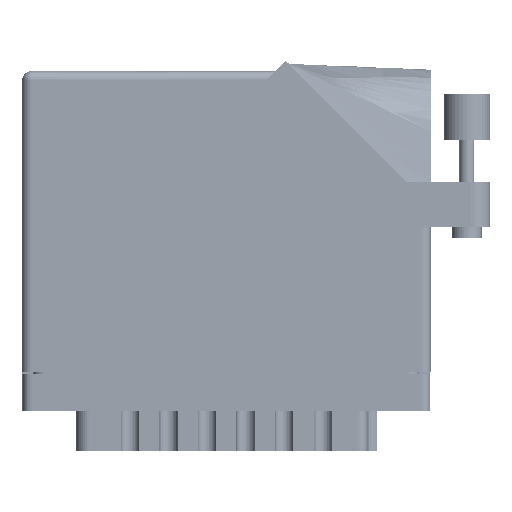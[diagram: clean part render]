
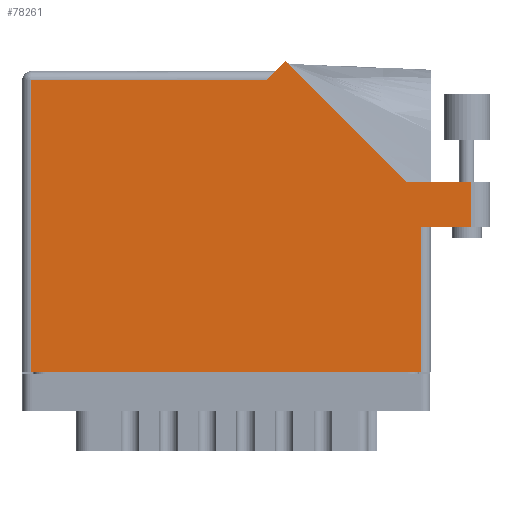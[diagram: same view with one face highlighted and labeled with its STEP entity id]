
A CAD part, front view. The second image highlights one B-rep face of the part: STEP entity #78261.
In plain terms, the highlighted face is planar.
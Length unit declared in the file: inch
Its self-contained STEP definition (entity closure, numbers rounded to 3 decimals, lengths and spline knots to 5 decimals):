
#1339 = CARTESIAN_POINT ( 'NONE',  ( 3.03, 1.287, 0. ) ) ;
#1963 = VECTOR ( 'NONE', #30588, 39.37008 ) ;
#4113 = VECTOR ( 'NONE', #65692, 39.37008 ) ;
#4821 = AXIS2_PLACEMENT_3D ( 'NONE', #58448, #73089, #73413 ) ;
#5466 = CARTESIAN_POINT ( 'NONE',  ( 2.755, 0.98, 0. ) ) ;
#5762 = CARTESIAN_POINT ( 'NONE',  ( 0., 0., 0. ) ) ;
#5935 = CARTESIAN_POINT ( 'NONE',  ( 0.062, 1.968, 0. ) ) ;
#6547 = ORIENTED_EDGE ( 'NONE', *, *, #66881, .T. ) ;
#8380 = LINE ( 'NONE', #1339, #60806 ) ;
#8432 = CARTESIAN_POINT ( 'NONE',  ( 0.062, 0., 0. ) ) ;
#10800 = ORIENTED_EDGE ( 'NONE', *, *, #62293, .T. ) ;
#11530 = VERTEX_POINT ( 'NONE', #52849 ) ;
#14372 = VECTOR ( 'NONE', #73338, 39.37008 ) ;
#14807 = LINE ( 'NONE', #8432, #29937 ) ;
#16790 = VERTEX_POINT ( 'NONE', #54575 ) ;
#17997 = VERTEX_POINT ( 'NONE', #92104 ) ;
#19635 = CARTESIAN_POINT ( 'NONE',  ( 3.03, 1.287, 0. ) ) ;
#21510 = EDGE_CURVE ( 'NONE', #16790, #96286, #39253, .T. ) ;
#23923 = EDGE_CURVE ( 'NONE', #17997, #40490, #8380, .T. ) ;
#25643 = DIRECTION ( 'NONE',  ( 0., -1., 0. ) ) ;
#29937 = VECTOR ( 'NONE', #25643, 39.37008 ) ;
#30588 = DIRECTION ( 'NONE',  ( -1., 0., 0. ) ) ;
#32725 = VECTOR ( 'NONE', #68590, 39.37008 ) ;
#38927 = CARTESIAN_POINT ( 'NONE',  ( 2.58942, 1.287, 0. ) ) ;
#39253 = LINE ( 'NONE', #75039, #55508 ) ;
#39541 = ORIENTED_EDGE ( 'NONE', *, *, #69104, .T. ) ;
#40005 = VERTEX_POINT ( 'NONE', #42595 ) ;
#40490 = VERTEX_POINT ( 'NONE', #19635 ) ;
#41667 = CARTESIAN_POINT ( 'NONE',  ( 1.77571, 2.10071, 0. ) ) ;
#42595 = CARTESIAN_POINT ( 'NONE',  ( 2.693, 0.98, 0. ) ) ;
#43759 = CARTESIAN_POINT ( 'NONE',  ( 1.705, 2.03, 0. ) ) ;
#45574 = CARTESIAN_POINT ( 'NONE',  ( 3.155, 1.287, 0. ) ) ;
#49593 = FACE_OUTER_BOUND ( 'NONE', #93399, .T. ) ;
#51939 = ORIENTED_EDGE ( 'NONE', *, *, #69536, .T. ) ;
#52575 = LINE ( 'NONE', #66388, #32725 ) ;
#52711 = VECTOR ( 'NONE', #80405, 39.37008 ) ;
#52849 = CARTESIAN_POINT ( 'NONE',  ( 2.693, 0., 0. ) ) ;
#54575 = CARTESIAN_POINT ( 'NONE',  ( 1.643, 1.968, 0. ) ) ;
#54868 = VERTEX_POINT ( 'NONE', #65681 ) ;
#55508 = VECTOR ( 'NONE', #90692, 39.37008 ) ;
#57042 = EDGE_CURVE ( 'NONE', #40005, #17997, #72498, .T. ) ;
#57803 = PLANE ( 'NONE',  #4821 ) ;
#58448 = CARTESIAN_POINT ( 'NONE',  ( 0., 2.03, 0. ) ) ;
#60655 = LINE ( 'NONE', #79170, #85193 ) ;
#60806 = VECTOR ( 'NONE', #76262, 39.37008 ) ;
#62293 = EDGE_CURVE ( 'NONE', #79389, #16790, #74983, .T. ) ;
#65681 = CARTESIAN_POINT ( 'NONE',  ( 0.062, 0., 0. ) ) ;
#65692 = DIRECTION ( 'NONE',  ( 1., 0., 0. ) ) ;
#66388 = CARTESIAN_POINT ( 'NONE',  ( 2.58942, 1.287, 0. ) ) ;
#66881 = EDGE_CURVE ( 'NONE', #87470, #79389, #52575, .T. ) ;
#66990 = EDGE_CURVE ( 'NONE', #11530, #40005, #60655, .T. ) ;
#68590 = DIRECTION ( 'NONE',  ( -0.707, 0.707, 0. ) ) ;
#69104 = EDGE_CURVE ( 'NONE', #40490, #87470, #73118, .T. ) ;
#69157 = EDGE_CURVE ( 'NONE', #96286, #54868, #14807, .T. ) ;
#69536 = EDGE_CURVE ( 'NONE', #54868, #11530, #79969, .T. ) ;
#72498 = LINE ( 'NONE', #5466, #52711 ) ;
#73089 = DIRECTION ( 'NONE',  ( 0., 0., -1. ) ) ;
#73118 = LINE ( 'NONE', #45574, #1963 ) ;
#73338 = DIRECTION ( 'NONE',  ( -0.707, -0.707, 0. ) ) ;
#73413 = DIRECTION ( 'NONE',  ( -1., 0., 0. ) ) ;
#73758 = ORIENTED_EDGE ( 'NONE', *, *, #69157, .T. ) ;
#74534 = ORIENTED_EDGE ( 'NONE', *, *, #21510, .T. ) ;
#74983 = LINE ( 'NONE', #43759, #14372 ) ;
#75039 = CARTESIAN_POINT ( 'NONE',  ( 0., 1.968, 0. ) ) ;
#75876 = ORIENTED_EDGE ( 'NONE', *, *, #57042, .T. ) ;
#76262 = DIRECTION ( 'NONE',  ( 0., 1., 0. ) ) ;
#78226 = ORIENTED_EDGE ( 'NONE', *, *, #66990, .T. ) ;
#78261 = ADVANCED_FACE ( 'NONE', ( #49593 ), #57803, .F. ) ;
#79170 = CARTESIAN_POINT ( 'NONE',  ( 2.693, 0.98, 0. ) ) ;
#79389 = VERTEX_POINT ( 'NONE', #41667 ) ;
#79969 = LINE ( 'NONE', #5762, #4113 ) ;
#80405 = DIRECTION ( 'NONE',  ( 1., 0., 0. ) ) ;
#82143 = ORIENTED_EDGE ( 'NONE', *, *, #23923, .T. ) ;
#85193 = VECTOR ( 'NONE', #85709, 39.37008 ) ;
#85709 = DIRECTION ( 'NONE',  ( 0., 1., 0. ) ) ;
#87470 = VERTEX_POINT ( 'NONE', #38927 ) ;
#90692 = DIRECTION ( 'NONE',  ( -1., 0., 0. ) ) ;
#92104 = CARTESIAN_POINT ( 'NONE',  ( 3.03, 0.98, 0. ) ) ;
#93399 = EDGE_LOOP ( 'NONE', ( #75876, #82143, #39541, #6547, #10800, #74534, #73758, #51939, #78226 ) ) ;
#96286 = VERTEX_POINT ( 'NONE', #5935 ) ;
